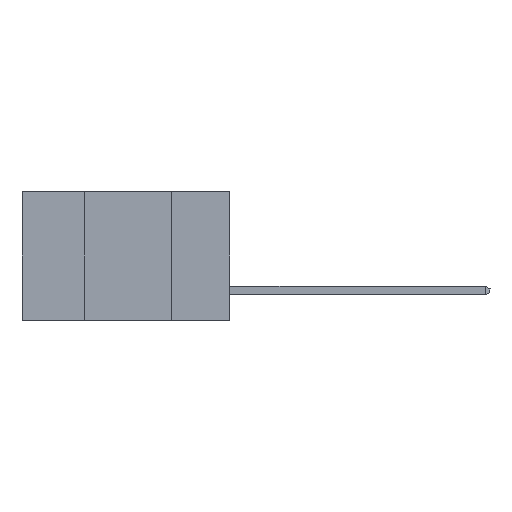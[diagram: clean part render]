
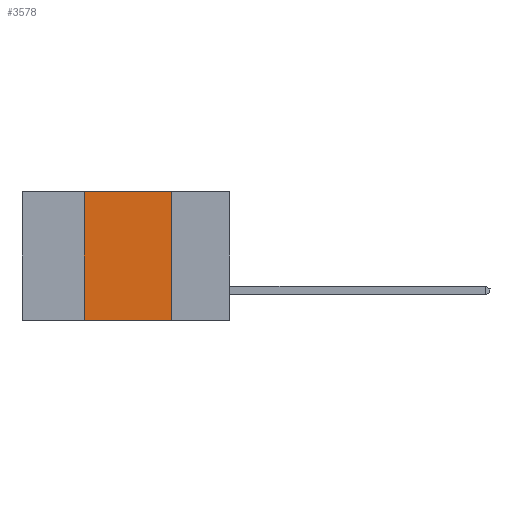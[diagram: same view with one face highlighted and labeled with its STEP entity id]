
A CAD part, left-side view. The second image highlights one B-rep face of the part: STEP entity #3578.
In plain terms, the highlighted planar face has unit normal (-1, 0, 0).
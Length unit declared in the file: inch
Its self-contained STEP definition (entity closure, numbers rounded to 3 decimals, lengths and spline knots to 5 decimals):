
#662 = DIRECTION ( 'NONE',  ( 1., 0., 0. ) ) ;
#1029 = ORIENTED_EDGE ( 'NONE', *, *, #9994, .F. ) ;
#1475 = EDGE_CURVE ( 'NONE', #7234, #10819, #11419, .T. ) ;
#2027 = VECTOR ( 'NONE', #9335, 39.37008 ) ;
#2273 = ORIENTED_EDGE ( 'NONE', *, *, #11922, .F. ) ;
#2885 = DIRECTION ( 'NONE',  ( 0., 0., -1. ) ) ;
#3188 = LINE ( 'NONE', #7474, #6159 ) ;
#3381 = EDGE_CURVE ( 'NONE', #8675, #10819, #7961, .T. ) ;
#3578 = ADVANCED_FACE ( 'NONE', ( #10418 ), #12483, .F. ) ;
#4779 = EDGE_LOOP ( 'NONE', ( #5865, #1029, #2273, #9825 ) ) ;
#5865 = ORIENTED_EDGE ( 'NONE', *, *, #3381, .F. ) ;
#6043 = CARTESIAN_POINT ( 'NONE',  ( 0., 0.6, 0. ) ) ;
#6064 = CARTESIAN_POINT ( 'NONE',  ( 0., 0.6, 0. ) ) ;
#6159 = VECTOR ( 'NONE', #11994, 39.37008 ) ;
#6940 = CARTESIAN_POINT ( 'NONE',  ( 0., 0.42, 0. ) ) ;
#7121 = VECTOR ( 'NONE', #11132, 39.37008 ) ;
#7234 = VERTEX_POINT ( 'NONE', #9941 ) ;
#7474 = CARTESIAN_POINT ( 'NONE',  ( 0., 0.42, -0.37 ) ) ;
#7961 = LINE ( 'NONE', #12277, #7121 ) ;
#8115 = VECTOR ( 'NONE', #9173, 39.37008 ) ;
#8341 = LINE ( 'NONE', #6064, #2027 ) ;
#8675 = VERTEX_POINT ( 'NONE', #9260 ) ;
#9173 = DIRECTION ( 'NONE',  ( 0., -1., 0. ) ) ;
#9260 = CARTESIAN_POINT ( 'NONE',  ( 0., 0.17, 0. ) ) ;
#9335 = DIRECTION ( 'NONE',  ( 0., -1., 0. ) ) ;
#9825 = ORIENTED_EDGE ( 'NONE', *, *, #1475, .T. ) ;
#9941 = CARTESIAN_POINT ( 'NONE',  ( 0., 0.42, -0.37 ) ) ;
#9994 = EDGE_CURVE ( 'NONE', #12473, #8675, #8341, .T. ) ;
#10418 = FACE_OUTER_BOUND ( 'NONE', #4779, .T. ) ;
#10819 = VERTEX_POINT ( 'NONE', #12273 ) ;
#11132 = DIRECTION ( 'NONE',  ( 0., 0., -1. ) ) ;
#11418 = AXIS2_PLACEMENT_3D ( 'NONE', #6043, #662, #2885 ) ;
#11419 = LINE ( 'NONE', #13550, #8115 ) ;
#11922 = EDGE_CURVE ( 'NONE', #7234, #12473, #3188, .T. ) ;
#11994 = DIRECTION ( 'NONE',  ( 0., 0., 1. ) ) ;
#12273 = CARTESIAN_POINT ( 'NONE',  ( 0., 0.17, -0.37 ) ) ;
#12277 = CARTESIAN_POINT ( 'NONE',  ( 0., 0.17, -0.37 ) ) ;
#12473 = VERTEX_POINT ( 'NONE', #6940 ) ;
#12483 = PLANE ( 'NONE',  #11418 ) ;
#13550 = CARTESIAN_POINT ( 'NONE',  ( 0., 0.6, -0.37 ) ) ;
